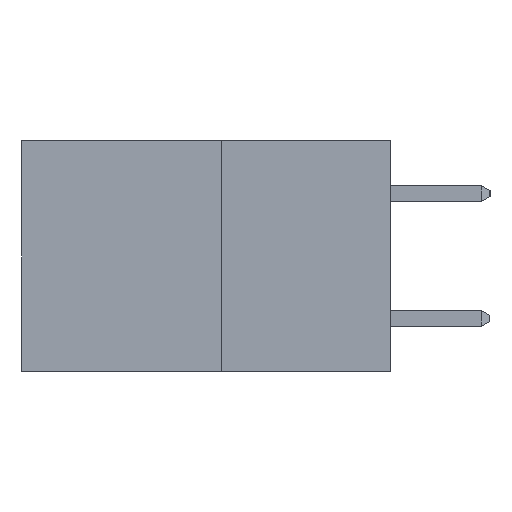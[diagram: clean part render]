
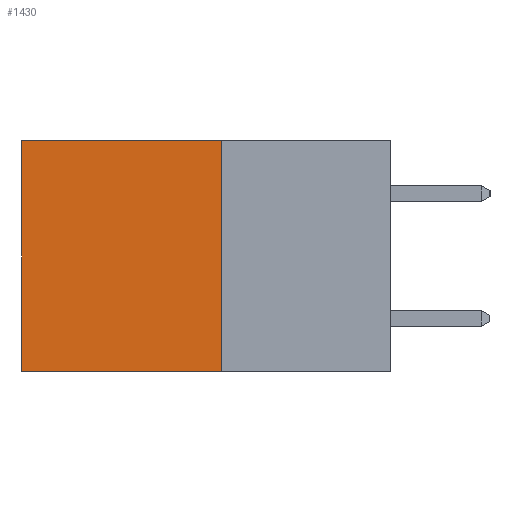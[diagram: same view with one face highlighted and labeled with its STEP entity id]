
A CAD part, left-side view. The second image highlights one B-rep face of the part: STEP entity #1430.
In plain terms, the highlighted planar face has unit normal (-1, 0, 0).
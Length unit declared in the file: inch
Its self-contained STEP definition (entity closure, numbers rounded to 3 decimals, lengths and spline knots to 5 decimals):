
#974 = VECTOR ( 'NONE', #981, 39.37008 ) ;
#981 = DIRECTION ( 'NONE',  ( 0., 1., 0. ) ) ;
#1430 = ADVANCED_FACE ( 'NONE', ( #5181 ), #21371, .F. ) ;
#1431 = ORIENTED_EDGE ( 'NONE', *, *, #2136, .T. ) ;
#2136 = EDGE_CURVE ( 'NONE', #23030, #16689, #5424, .T. ) ;
#2338 = AXIS2_PLACEMENT_3D ( 'NONE', #20901, #20860, #20825 ) ;
#2532 = CARTESIAN_POINT ( 'NONE',  ( 0.277, 0.27, 0. ) ) ;
#2670 = VECTOR ( 'NONE', #15491, 39.37008 ) ;
#2942 = VERTEX_POINT ( 'NONE', #13013 ) ;
#3255 = LINE ( 'NONE', #8243, #2670 ) ;
#3334 = ORIENTED_EDGE ( 'NONE', *, *, #20503, .F. ) ;
#4518 = CARTESIAN_POINT ( 'NONE',  ( 0.277, 0.59, -0.37 ) ) ;
#5181 = FACE_OUTER_BOUND ( 'NONE', #9742, .T. ) ;
#5395 = LINE ( 'NONE', #8103, #19293 ) ;
#5424 = LINE ( 'NONE', #2532, #974 ) ;
#5525 = CARTESIAN_POINT ( 'NONE',  ( 0.277, 0.59, -0.37 ) ) ;
#8103 = CARTESIAN_POINT ( 'NONE',  ( 0.277, 0.27, -0.37 ) ) ;
#8243 = CARTESIAN_POINT ( 'NONE',  ( 0.277, 0.27, -0.37 ) ) ;
#9742 = EDGE_LOOP ( 'NONE', ( #16363, #15747, #3334, #1431 ) ) ;
#11550 = CARTESIAN_POINT ( 'NONE',  ( 0.277, 0.27, 0. ) ) ;
#11638 = EDGE_CURVE ( 'NONE', #2942, #18608, #3255, .T. ) ;
#12209 = LINE ( 'NONE', #5525, #12765 ) ;
#12765 = VECTOR ( 'NONE', #18248, 39.37008 ) ;
#12814 = CARTESIAN_POINT ( 'NONE',  ( 0.277, 0.59, 0. ) ) ;
#13013 = CARTESIAN_POINT ( 'NONE',  ( 0.277, 0.27, -0.37 ) ) ;
#15326 = EDGE_CURVE ( 'NONE', #16689, #18608, #12209, .T. ) ;
#15354 = DIRECTION ( 'NONE',  ( 0., 0., -1. ) ) ;
#15491 = DIRECTION ( 'NONE',  ( 0., 1., 0. ) ) ;
#15747 = ORIENTED_EDGE ( 'NONE', *, *, #11638, .F. ) ;
#16363 = ORIENTED_EDGE ( 'NONE', *, *, #15326, .T. ) ;
#16689 = VERTEX_POINT ( 'NONE', #12814 ) ;
#18248 = DIRECTION ( 'NONE',  ( 0., 0., -1. ) ) ;
#18608 = VERTEX_POINT ( 'NONE', #4518 ) ;
#19293 = VECTOR ( 'NONE', #15354, 39.37008 ) ;
#20503 = EDGE_CURVE ( 'NONE', #23030, #2942, #5395, .T. ) ;
#20825 = DIRECTION ( 'NONE',  ( 0., 0., -1. ) ) ;
#20860 = DIRECTION ( 'NONE',  ( 1., 0., 0. ) ) ;
#20901 = CARTESIAN_POINT ( 'NONE',  ( 0.277, 0.27, -0.37 ) ) ;
#21371 = PLANE ( 'NONE',  #2338 ) ;
#23030 = VERTEX_POINT ( 'NONE', #11550 ) ;
